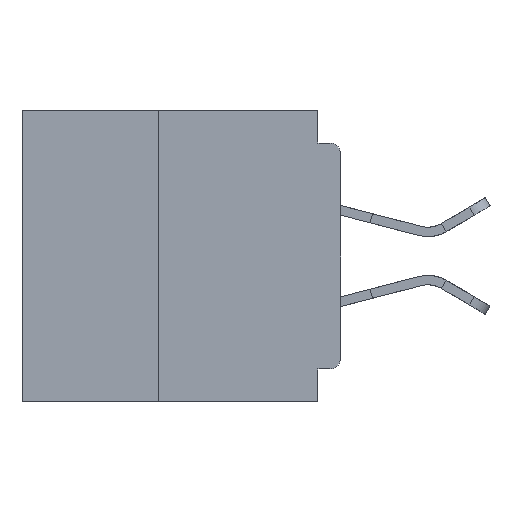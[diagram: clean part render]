
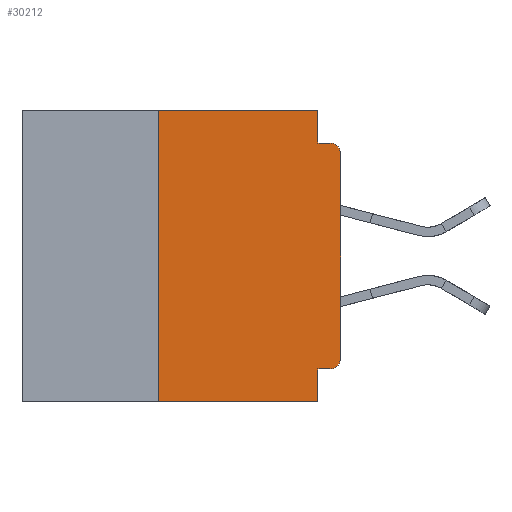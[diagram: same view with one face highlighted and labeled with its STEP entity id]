
A CAD part, left-side view. The second image highlights one B-rep face of the part: STEP entity #30212.
In plain terms, the highlighted planar face has unit normal (-1, 0, 0).
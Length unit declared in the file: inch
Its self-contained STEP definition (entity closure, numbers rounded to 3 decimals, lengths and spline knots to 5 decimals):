
#1083 = LINE ( 'NONE', #36552, #10207 ) ;
#1326 = VERTEX_POINT ( 'NONE', #23515 ) ;
#2805 = DIRECTION ( 'NONE',  ( 0., 0., -1. ) ) ;
#3464 = CARTESIAN_POINT ( 'NONE',  ( 0., 0.015, -0.355 ) ) ;
#3656 = ORIENTED_EDGE ( 'NONE', *, *, #35651, .T. ) ;
#4352 = CIRCLE ( 'NONE', #38102, 0.015 ) ;
#4759 = ORIENTED_EDGE ( 'NONE', *, *, #12591, .T. ) ;
#4960 = CARTESIAN_POINT ( 'NONE',  ( 0., 0., -0.06 ) ) ;
#5087 = ORIENTED_EDGE ( 'NONE', *, *, #11942, .F. ) ;
#5694 = VECTOR ( 'NONE', #23590, 39.37008 ) ;
#5744 = LINE ( 'NONE', #39793, #39608 ) ;
#6050 = ORIENTED_EDGE ( 'NONE', *, *, #9192, .T. ) ;
#7573 = EDGE_CURVE ( 'NONE', #28275, #42129, #35623, .T. ) ;
#8784 = EDGE_CURVE ( 'NONE', #21305, #27886, #9051, .T. ) ;
#9051 = LINE ( 'NONE', #26312, #26129 ) ;
#9192 = EDGE_CURVE ( 'NONE', #21305, #42129, #43804, .T. ) ;
#9519 = AXIS2_PLACEMENT_3D ( 'NONE', #38334, #18192, #41678 ) ;
#10207 = VECTOR ( 'NONE', #43241, 39.37008 ) ;
#11369 = DIRECTION ( 'NONE',  ( -1., 0., 0. ) ) ;
#11942 = EDGE_CURVE ( 'NONE', #27886, #1326, #1083, .T. ) ;
#12591 = EDGE_CURVE ( 'NONE', #17331, #30523, #27789, .T. ) ;
#12606 = DIRECTION ( 'NONE',  ( 0., 0., -1. ) ) ;
#12862 = LINE ( 'NONE', #28764, #29937 ) ;
#14146 = DIRECTION ( 'NONE',  ( 0., 0., 1. ) ) ;
#14553 = CARTESIAN_POINT ( 'NONE',  ( 0., 0.015, -0.045 ) ) ;
#14570 = VECTOR ( 'NONE', #14146, 39.37008 ) ;
#14762 = LINE ( 'NONE', #43581, #5694 ) ;
#14846 = AXIS2_PLACEMENT_3D ( 'NONE', #19854, #23273, #2805 ) ;
#15212 = DIRECTION ( 'NONE',  ( 0., 1., 0. ) ) ;
#15945 = CARTESIAN_POINT ( 'NONE',  ( 0., 0.031, -0.4 ) ) ;
#16166 = DIRECTION ( 'NONE',  ( 0., 0., 1. ) ) ;
#16404 = CARTESIAN_POINT ( 'NONE',  ( 0., 0.031, -0.355 ) ) ;
#17331 = VERTEX_POINT ( 'NONE', #3464 ) ;
#18192 = DIRECTION ( 'NONE',  ( -1., 0., 0. ) ) ;
#18370 = CARTESIAN_POINT ( 'NONE',  ( 0., 0.437, -0.4 ) ) ;
#19438 = EDGE_CURVE ( 'NONE', #1326, #32458, #5744, .T. ) ;
#19854 = CARTESIAN_POINT ( 'NONE',  ( 0., 0.437, 0. ) ) ;
#21305 = VERTEX_POINT ( 'NONE', #41467 ) ;
#22098 = ORIENTED_EDGE ( 'NONE', *, *, #43411, .F. ) ;
#23273 = DIRECTION ( 'NONE',  ( 1., 0., 0. ) ) ;
#23515 = CARTESIAN_POINT ( 'NONE',  ( 0., 0.031, 0. ) ) ;
#23590 = DIRECTION ( 'NONE',  ( 0., -1., 0. ) ) ;
#24973 = EDGE_CURVE ( 'NONE', #32458, #29081, #14762, .T. ) ;
#25096 = DIRECTION ( 'NONE',  ( 0., -1., 0. ) ) ;
#25496 = ORIENTED_EDGE ( 'NONE', *, *, #8784, .F. ) ;
#26087 = VECTOR ( 'NONE', #25096, 39.37008 ) ;
#26129 = VECTOR ( 'NONE', #16166, 39.37008 ) ;
#26312 = CARTESIAN_POINT ( 'NONE',  ( 0., 0.25, -0.4 ) ) ;
#26528 = VERTEX_POINT ( 'NONE', #4960 ) ;
#26790 = VECTOR ( 'NONE', #42844, 39.37008 ) ;
#27789 = CIRCLE ( 'NONE', #9519, 0.015 ) ;
#27886 = VERTEX_POINT ( 'NONE', #31427 ) ;
#28275 = VERTEX_POINT ( 'NONE', #16404 ) ;
#28764 = CARTESIAN_POINT ( 'NONE',  ( 0., 0., -0.355 ) ) ;
#28887 = CARTESIAN_POINT ( 'NONE',  ( 0., 0.031, -0.045 ) ) ;
#29081 = VERTEX_POINT ( 'NONE', #14553 ) ;
#29937 = VECTOR ( 'NONE', #15212, 39.37008 ) ;
#30212 = ADVANCED_FACE ( 'NONE', ( #41974 ), #43285, .F. ) ;
#30412 = EDGE_CURVE ( 'NONE', #30523, #26528, #32596, .T. ) ;
#30498 = EDGE_LOOP ( 'NONE', ( #35697, #3656, #39652, #42867, #5087, #25496, #6050, #30697, #22098, #4759 ) ) ;
#30523 = VERTEX_POINT ( 'NONE', #31516 ) ;
#30697 = ORIENTED_EDGE ( 'NONE', *, *, #7573, .F. ) ;
#31427 = CARTESIAN_POINT ( 'NONE',  ( 0., 0.25, 0. ) ) ;
#31516 = CARTESIAN_POINT ( 'NONE',  ( 0., 0., -0.34 ) ) ;
#31725 = CARTESIAN_POINT ( 'NONE',  ( 0., 0.015, -0.06 ) ) ;
#32458 = VERTEX_POINT ( 'NONE', #28887 ) ;
#32596 = LINE ( 'NONE', #37755, #14570 ) ;
#35056 = DIRECTION ( 'NONE',  ( 0., 0., -1. ) ) ;
#35114 = CARTESIAN_POINT ( 'NONE',  ( 0., 0.031, -0.4 ) ) ;
#35623 = LINE ( 'NONE', #15945, #26790 ) ;
#35651 = EDGE_CURVE ( 'NONE', #26528, #29081, #4352, .T. ) ;
#35697 = ORIENTED_EDGE ( 'NONE', *, *, #30412, .T. ) ;
#36552 = CARTESIAN_POINT ( 'NONE',  ( 0., 0.437, 0. ) ) ;
#37755 = CARTESIAN_POINT ( 'NONE',  ( 0., 0., 0. ) ) ;
#38102 = AXIS2_PLACEMENT_3D ( 'NONE', #31725, #11369, #35056 ) ;
#38334 = CARTESIAN_POINT ( 'NONE',  ( 0., 0.015, -0.34 ) ) ;
#39608 = VECTOR ( 'NONE', #12606, 39.37008 ) ;
#39652 = ORIENTED_EDGE ( 'NONE', *, *, #24973, .F. ) ;
#39793 = CARTESIAN_POINT ( 'NONE',  ( 0., 0.031, 0. ) ) ;
#41467 = CARTESIAN_POINT ( 'NONE',  ( 0., 0.25, -0.4 ) ) ;
#41678 = DIRECTION ( 'NONE',  ( 0., 0., -1. ) ) ;
#41974 = FACE_OUTER_BOUND ( 'NONE', #30498, .T. ) ;
#42129 = VERTEX_POINT ( 'NONE', #35114 ) ;
#42844 = DIRECTION ( 'NONE',  ( 0., 0., -1. ) ) ;
#42867 = ORIENTED_EDGE ( 'NONE', *, *, #19438, .F. ) ;
#43241 = DIRECTION ( 'NONE',  ( 0., -1., 0. ) ) ;
#43285 = PLANE ( 'NONE',  #14846 ) ;
#43411 = EDGE_CURVE ( 'NONE', #17331, #28275, #12862, .T. ) ;
#43581 = CARTESIAN_POINT ( 'NONE',  ( 0., 0., -0.045 ) ) ;
#43804 = LINE ( 'NONE', #18370, #26087 ) ;
